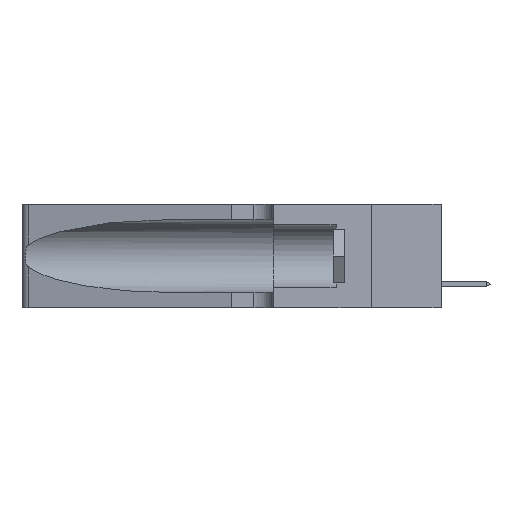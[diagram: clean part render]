
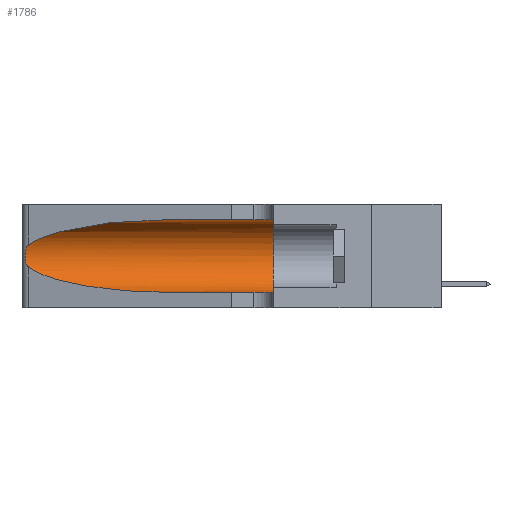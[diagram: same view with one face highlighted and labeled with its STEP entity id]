
A CAD part, left-side view. The second image highlights one B-rep face of the part: STEP entity #1786.
In plain terms, the highlighted cylindrical face has radius 3.308 mm (diameter 6.617 mm), a partial arc.
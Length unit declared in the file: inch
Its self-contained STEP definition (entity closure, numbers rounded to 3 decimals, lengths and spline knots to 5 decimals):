
#1786 = ADVANCED_FACE ( 'NONE', ( #18276 ), #19081, .F. ) ;
#1891 = CARTESIAN_POINT ( 'NONE',  ( 0.25487, 1.22718, 0.22369 ) ) ;
#1939 =( BOUNDED_CURVE ( )  B_SPLINE_CURVE ( 3, ( #3462, #31141, #30322, #28153 ),
 .UNSPECIFIED., .F., .F. ) 
 B_SPLINE_CURVE_WITH_KNOTS ( ( 4, 4 ),
 ( 3.44316, 4.71239 ),
 .UNSPECIFIED. ) 
 CURVE ( )  GEOMETRIC_REPRESENTATION_ITEM ( )  RATIONAL_B_SPLINE_CURVE ( ( 1., 0.87, 0.87, 1. ) ) 
 REPRESENTATION_ITEM ( '' )  );
#1952 = CARTESIAN_POINT ( 'NONE',  ( 0.25856, 1.23593, 0.16098 ) ) ;
#2331 = EDGE_CURVE ( 'NONE', #21953, #11761, #11441, .T. ) ;
#2359 = CARTESIAN_POINT ( 'NONE',  ( 0.25789, 1.23486, 0.15765 ) ) ;
#3180 = CARTESIAN_POINT ( 'NONE',  ( 0.1305, 1.61858, 0.31525 ) ) ;
#3271 = EDGE_CURVE ( 'NONE', #22166, #16679, #22759, .T. ) ;
#3462 = CARTESIAN_POINT ( 'NONE',  ( 0.25487, 1.22718, 0.14631 ) ) ;
#4588 = AXIS2_PLACEMENT_3D ( 'NONE', #6725, #19410, #19188 ) ;
#4757 = CARTESIAN_POINT ( 'NONE',  ( 0.26075, 1.23896, 0.19203 ) ) ;
#5702 = B_SPLINE_CURVE_WITH_KNOTS ( 'NONE', 3,
 ( #23644, #8878, #31134, #25991, #31245, #19284, #4757, #14604, #9714, #1952, #2359, #29311, #17186, #22029 ),
 .UNSPECIFIED., .F., .F.,
 ( 4, 2, 2, 2, 2, 2, 4 ),
 ( 0., 0.00027, 0.00053, 0.00107, 0.0016, 0.00187, 0.00214 ),
 .UNSPECIFIED. ) ;
#5871 = CIRCLE ( 'NONE', #4588, 0.13025 ) ;
#6725 = CARTESIAN_POINT ( 'NONE',  ( 0.1305, 0.35, 0.185 ) ) ;
#8440 = ORIENTED_EDGE ( 'NONE', *, *, #3271, .T. ) ;
#8655 = CARTESIAN_POINT ( 'NONE',  ( 0.1305, 0.35, 0.05475 ) ) ;
#8713 = EDGE_LOOP ( 'NONE', ( #26885, #10508, #17450, #8440, #29810, #31970 ) ) ;
#8878 = CARTESIAN_POINT ( 'NONE',  ( 0.25555, 1.22994, 0.2215 ) ) ;
#9714 = CARTESIAN_POINT ( 'NONE',  ( 0.26017, 1.23833, 0.17102 ) ) ;
#10263 = EDGE_CURVE ( 'NONE', #31491, #22166, #1939, .T. ) ;
#10508 = ORIENTED_EDGE ( 'NONE', *, *, #20905, .T. ) ;
#11441 =( BOUNDED_CURVE ( )  B_SPLINE_CURVE ( 3, ( #27210, #21960, #29950, #28711 ),
 .UNSPECIFIED., .F., .T. ) 
 B_SPLINE_CURVE_WITH_KNOTS ( ( 4, 4 ),
 ( 1.5708, 2.84003 ),
 .UNSPECIFIED. ) 
 CURVE ( )  GEOMETRIC_REPRESENTATION_ITEM ( )  RATIONAL_B_SPLINE_CURVE ( ( 1., 0.87, 0.87, 1. ) ) 
 REPRESENTATION_ITEM ( '' )  );
#11598 = CARTESIAN_POINT ( 'NONE',  ( 0.1305, 0.35, 0.31525 ) ) ;
#11761 = VERTEX_POINT ( 'NONE', #1891 ) ;
#14092 = VERTEX_POINT ( 'NONE', #11598 ) ;
#14130 = CARTESIAN_POINT ( 'NONE',  ( 0.1305, 0.72297, 0.31525 ) ) ;
#14604 = CARTESIAN_POINT ( 'NONE',  ( 0.26075, 1.23896, 0.178 ) ) ;
#15074 = DIRECTION ( 'NONE',  ( 0., 0., -1. ) ) ;
#16029 = CARTESIAN_POINT ( 'NONE',  ( 0.1305, 1.61858, 0.05475 ) ) ;
#16679 = VERTEX_POINT ( 'NONE', #8655 ) ;
#16954 = EDGE_CURVE ( 'NONE', #14092, #16679, #5871, .T. ) ;
#17186 = CARTESIAN_POINT ( 'NONE',  ( 0.25555, 1.22993, 0.14849 ) ) ;
#17450 = ORIENTED_EDGE ( 'NONE', *, *, #10263, .T. ) ;
#18276 = FACE_OUTER_BOUND ( 'NONE', #8713, .T. ) ;
#19081 = CYLINDRICAL_SURFACE ( 'NONE', #22807, 0.13025 ) ;
#19188 = DIRECTION ( 'NONE',  ( 0., 0., 1. ) ) ;
#19284 = CARTESIAN_POINT ( 'NONE',  ( 0.26018, 1.23835, 0.19895 ) ) ;
#19410 = DIRECTION ( 'NONE',  ( 0., 1., 0. ) ) ;
#19421 = CARTESIAN_POINT ( 'NONE',  ( 0.25487, 1.22718, 0.14631 ) ) ;
#20905 = EDGE_CURVE ( 'NONE', #11761, #31491, #5702, .T. ) ;
#21691 = VECTOR ( 'NONE', #23654, 39.37008 ) ;
#21953 = VERTEX_POINT ( 'NONE', #14130 ) ;
#21960 = CARTESIAN_POINT ( 'NONE',  ( 0.18966, 0.96281, 0.31525 ) ) ;
#21966 = CARTESIAN_POINT ( 'NONE',  ( 0.1305, 0.72297, 0.05475 ) ) ;
#22029 = CARTESIAN_POINT ( 'NONE',  ( 0.25487, 1.22718, 0.14631 ) ) ;
#22166 = VERTEX_POINT ( 'NONE', #21966 ) ;
#22759 = LINE ( 'NONE', #16029, #21691 ) ;
#22807 = AXIS2_PLACEMENT_3D ( 'NONE', #29790, #24557, #15074 ) ;
#23644 = CARTESIAN_POINT ( 'NONE',  ( 0.25487, 1.22718, 0.22369 ) ) ;
#23654 = DIRECTION ( 'NONE',  ( 0., -1., 0. ) ) ;
#24444 = EDGE_CURVE ( 'NONE', #21953, #14092, #29546, .T. ) ;
#24557 = DIRECTION ( 'NONE',  ( 0., -1., 0. ) ) ;
#25712 = DIRECTION ( 'NONE',  ( 0., -1., 0. ) ) ;
#25991 = CARTESIAN_POINT ( 'NONE',  ( 0.25787, 1.23484, 0.2124 ) ) ;
#26885 = ORIENTED_EDGE ( 'NONE', *, *, #2331, .T. ) ;
#27210 = CARTESIAN_POINT ( 'NONE',  ( 0.1305, 0.72297, 0.31525 ) ) ;
#27561 = VECTOR ( 'NONE', #25712, 39.37008 ) ;
#28153 = CARTESIAN_POINT ( 'NONE',  ( 0.1305, 0.72297, 0.05475 ) ) ;
#28711 = CARTESIAN_POINT ( 'NONE',  ( 0.25487, 1.22718, 0.22369 ) ) ;
#29311 = CARTESIAN_POINT ( 'NONE',  ( 0.25639, 1.23186, 0.15144 ) ) ;
#29546 = LINE ( 'NONE', #3180, #27561 ) ;
#29790 = CARTESIAN_POINT ( 'NONE',  ( 0.1305, 1.61858, 0.185 ) ) ;
#29810 = ORIENTED_EDGE ( 'NONE', *, *, #16954, .F. ) ;
#29950 = CARTESIAN_POINT ( 'NONE',  ( 0.2373, 1.15595, 0.28018 ) ) ;
#30322 = CARTESIAN_POINT ( 'NONE',  ( 0.18966, 0.96281, 0.05475 ) ) ;
#31134 = CARTESIAN_POINT ( 'NONE',  ( 0.25639, 1.23184, 0.21858 ) ) ;
#31141 = CARTESIAN_POINT ( 'NONE',  ( 0.2373, 1.15595, 0.08982 ) ) ;
#31245 = CARTESIAN_POINT ( 'NONE',  ( 0.25854, 1.2359, 0.20912 ) ) ;
#31491 = VERTEX_POINT ( 'NONE', #19421 ) ;
#31970 = ORIENTED_EDGE ( 'NONE', *, *, #24444, .F. ) ;
